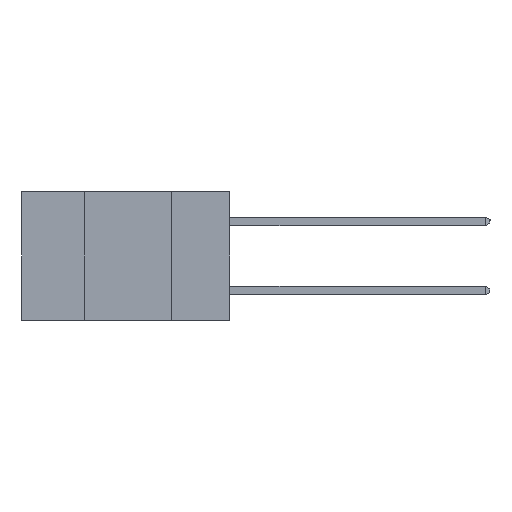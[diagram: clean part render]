
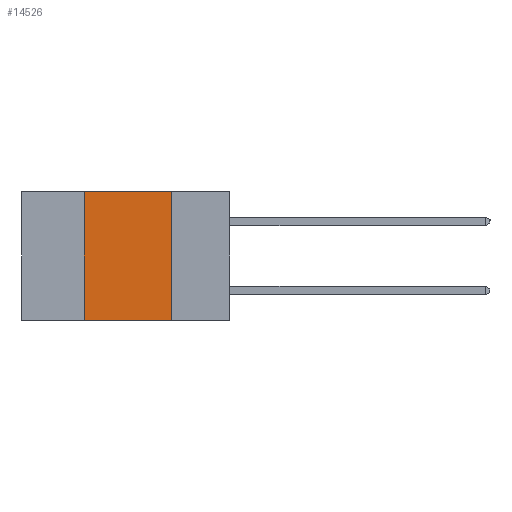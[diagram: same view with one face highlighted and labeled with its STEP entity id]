
A CAD part, left-side view. The second image highlights one B-rep face of the part: STEP entity #14526.
In plain terms, the highlighted planar face has unit normal (-1, 0, 0).
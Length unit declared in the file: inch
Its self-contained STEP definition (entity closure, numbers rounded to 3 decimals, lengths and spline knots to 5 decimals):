
#151 = CARTESIAN_POINT ( 'NONE',  ( 0., 0.6, -0.37 ) ) ;
#1412 = CARTESIAN_POINT ( 'NONE',  ( 0., 0.42, 0. ) ) ;
#1920 = CARTESIAN_POINT ( 'NONE',  ( 0., 0.6, 0. ) ) ;
#2676 = CARTESIAN_POINT ( 'NONE',  ( 0., 0.17, 0. ) ) ;
#3069 = EDGE_CURVE ( 'NONE', #10192, #9389, #15426, .T. ) ;
#3306 = LINE ( 'NONE', #8121, #4010 ) ;
#3396 = ORIENTED_EDGE ( 'NONE', *, *, #4031, .F. ) ;
#3958 = LINE ( 'NONE', #8746, #4825 ) ;
#4010 = VECTOR ( 'NONE', #10960, 39.37008 ) ;
#4031 = EDGE_CURVE ( 'NONE', #6353, #10192, #3958, .T. ) ;
#4340 = ORIENTED_EDGE ( 'NONE', *, *, #8553, .F. ) ;
#4825 = VECTOR ( 'NONE', #13622, 39.37008 ) ;
#6027 = ORIENTED_EDGE ( 'NONE', *, *, #8880, .T. ) ;
#6353 = VERTEX_POINT ( 'NONE', #14697 ) ;
#6758 = AXIS2_PLACEMENT_3D ( 'NONE', #11404, #15074, #10376 ) ;
#7222 = EDGE_LOOP ( 'NONE', ( #4340, #15435, #3396, #6027 ) ) ;
#7437 = DIRECTION ( 'NONE',  ( 0., -1., 0. ) ) ;
#7831 = FACE_OUTER_BOUND ( 'NONE', #7222, .T. ) ;
#8121 = CARTESIAN_POINT ( 'NONE',  ( 0., 0.17, -0.37 ) ) ;
#8553 = EDGE_CURVE ( 'NONE', #9389, #12021, #3306, .T. ) ;
#8746 = CARTESIAN_POINT ( 'NONE',  ( 0., 0.42, -0.37 ) ) ;
#8880 = EDGE_CURVE ( 'NONE', #6353, #12021, #12610, .T. ) ;
#9389 = VERTEX_POINT ( 'NONE', #2676 ) ;
#10192 = VERTEX_POINT ( 'NONE', #1412 ) ;
#10376 = DIRECTION ( 'NONE',  ( 0., 0., -1. ) ) ;
#10659 = VECTOR ( 'NONE', #7437, 39.37008 ) ;
#10960 = DIRECTION ( 'NONE',  ( 0., 0., -1. ) ) ;
#11404 = CARTESIAN_POINT ( 'NONE',  ( 0., 0.6, 0. ) ) ;
#11777 = CARTESIAN_POINT ( 'NONE',  ( 0., 0.17, -0.37 ) ) ;
#12021 = VERTEX_POINT ( 'NONE', #11777 ) ;
#12610 = LINE ( 'NONE', #151, #10659 ) ;
#12718 = DIRECTION ( 'NONE',  ( 0., -1., 0. ) ) ;
#13414 = VECTOR ( 'NONE', #12718, 39.37008 ) ;
#13622 = DIRECTION ( 'NONE',  ( 0., 0., 1. ) ) ;
#14526 = ADVANCED_FACE ( 'NONE', ( #7831 ), #15151, .F. ) ;
#14697 = CARTESIAN_POINT ( 'NONE',  ( 0., 0.42, -0.37 ) ) ;
#15074 = DIRECTION ( 'NONE',  ( 1., 0., 0. ) ) ;
#15151 = PLANE ( 'NONE',  #6758 ) ;
#15426 = LINE ( 'NONE', #1920, #13414 ) ;
#15435 = ORIENTED_EDGE ( 'NONE', *, *, #3069, .F. ) ;
